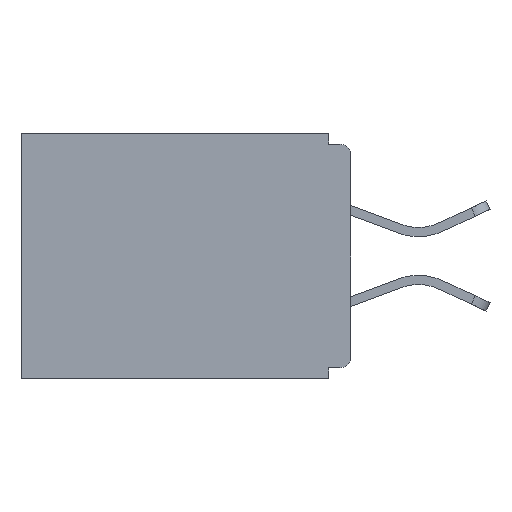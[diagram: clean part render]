
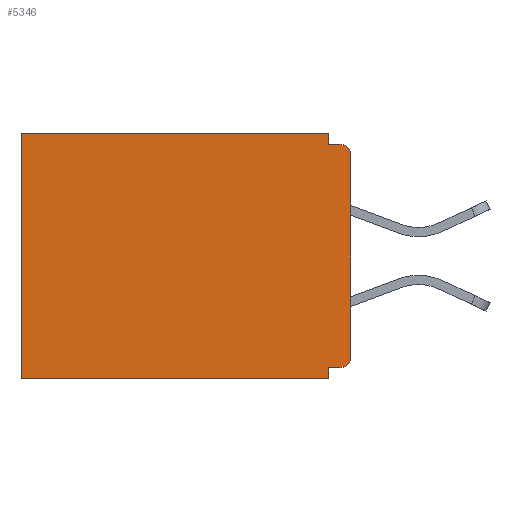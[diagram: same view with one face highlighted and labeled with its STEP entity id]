
A CAD part, left-side view. The second image highlights one B-rep face of the part: STEP entity #5346.
In plain terms, the highlighted planar face has unit normal (-1, 0, 0).
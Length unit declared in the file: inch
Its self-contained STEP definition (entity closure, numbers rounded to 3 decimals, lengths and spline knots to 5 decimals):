
#561 = CARTESIAN_POINT ( 'NONE',  ( 0.298, 0., -0.03 ) ) ;
#940 = VERTEX_POINT ( 'NONE', #1920 ) ;
#970 = VECTOR ( 'NONE', #1471, 39.37008 ) ;
#1181 = DIRECTION ( 'NONE',  ( 0., 0., -1. ) ) ;
#1192 = CARTESIAN_POINT ( 'NONE',  ( 0.298, 0.015, -0.015 ) ) ;
#1256 = DIRECTION ( 'NONE',  ( 0., 0., -1. ) ) ;
#1259 = DIRECTION ( 'NONE',  ( 0., -1., 0. ) ) ;
#1322 = VECTOR ( 'NONE', #5006, 39.37008 ) ;
#1471 = DIRECTION ( 'NONE',  ( 0., 0., -1. ) ) ;
#1920 = CARTESIAN_POINT ( 'NONE',  ( 0.298, 0., -0.313 ) ) ;
#2230 = AXIS2_PLACEMENT_3D ( 'NONE', #13511, #8339, #1256 ) ;
#2332 = EDGE_LOOP ( 'NONE', ( #15983, #18313, #9419, #7935, #17134, #21832, #17767, #9059, #19388, #3299 ) ) ;
#2635 = EDGE_CURVE ( 'NONE', #10745, #18288, #10756, .T. ) ;
#3299 = ORIENTED_EDGE ( 'NONE', *, *, #9171, .F. ) ;
#3429 = DIRECTION ( 'NONE',  ( 0., 0., -1. ) ) ;
#3527 = FACE_OUTER_BOUND ( 'NONE', #2332, .T. ) ;
#3716 = VECTOR ( 'NONE', #15571, 39.37008 ) ;
#3941 = CARTESIAN_POINT ( 'NONE',  ( 0.298, 0.46, -0.343 ) ) ;
#4292 = CARTESIAN_POINT ( 'NONE',  ( 0.298, 0.031, -0.343 ) ) ;
#4934 = CARTESIAN_POINT ( 'NONE',  ( 0.298, 0.015, -0.03 ) ) ;
#4982 = CIRCLE ( 'NONE', #10778, 0.015 ) ;
#5006 = DIRECTION ( 'NONE',  ( 0., 1., 0. ) ) ;
#5346 = ADVANCED_FACE ( 'NONE', ( #3527 ), #20271, .F. ) ;
#5601 = VECTOR ( 'NONE', #10202, 39.37008 ) ;
#5848 = LINE ( 'NONE', #20559, #5601 ) ;
#6840 = CARTESIAN_POINT ( 'NONE',  ( 0.298, 0., 0. ) ) ;
#7559 = LINE ( 'NONE', #6840, #11602 ) ;
#7646 = VERTEX_POINT ( 'NONE', #9323 ) ;
#7935 = ORIENTED_EDGE ( 'NONE', *, *, #17537, .T. ) ;
#8339 = DIRECTION ( 'NONE',  ( 1., 0., 0. ) ) ;
#8606 = CARTESIAN_POINT ( 'NONE',  ( 0.298, 0.031, -0.343 ) ) ;
#8850 = CARTESIAN_POINT ( 'NONE',  ( 0.298, 0.031, -0.015 ) ) ;
#9059 = ORIENTED_EDGE ( 'NONE', *, *, #17984, .F. ) ;
#9065 = LINE ( 'NONE', #11633, #970 ) ;
#9171 = EDGE_CURVE ( 'NONE', #16404, #940, #9065, .T. ) ;
#9214 = CIRCLE ( 'NONE', #11218, 0.015 ) ;
#9238 = DIRECTION ( 'NONE',  ( 0., 0., -1. ) ) ;
#9320 = VECTOR ( 'NONE', #9238, 39.37008 ) ;
#9323 = CARTESIAN_POINT ( 'NONE',  ( 0.298, 0.031, -0.328 ) ) ;
#9419 = ORIENTED_EDGE ( 'NONE', *, *, #13753, .F. ) ;
#10105 = DIRECTION ( 'NONE',  ( 0., 1., 0. ) ) ;
#10187 = EDGE_CURVE ( 'NONE', #7646, #10433, #12568, .T. ) ;
#10202 = DIRECTION ( 'NONE',  ( 0., 1., 0. ) ) ;
#10298 = CARTESIAN_POINT ( 'NONE',  ( 0.298, 0.031, 0. ) ) ;
#10433 = VERTEX_POINT ( 'NONE', #8606 ) ;
#10745 = VERTEX_POINT ( 'NONE', #20727 ) ;
#10756 = LINE ( 'NONE', #13740, #3716 ) ;
#10778 = AXIS2_PLACEMENT_3D ( 'NONE', #20349, #13433, #1181 ) ;
#11218 = AXIS2_PLACEMENT_3D ( 'NONE', #4934, #13816, #3429 ) ;
#11602 = VECTOR ( 'NONE', #10105, 39.37008 ) ;
#11633 = CARTESIAN_POINT ( 'NONE',  ( 0.298, 0., 0. ) ) ;
#12568 = LINE ( 'NONE', #4292, #9320 ) ;
#13433 = DIRECTION ( 'NONE',  ( -1., 0., 0. ) ) ;
#13511 = CARTESIAN_POINT ( 'NONE',  ( 0.298, 0., 0. ) ) ;
#13696 = VERTEX_POINT ( 'NONE', #8850 ) ;
#13740 = CARTESIAN_POINT ( 'NONE',  ( 0.298, 0.46, 0. ) ) ;
#13753 = EDGE_CURVE ( 'NONE', #21129, #13696, #17536, .T. ) ;
#13816 = DIRECTION ( 'NONE',  ( -1., 0., 0. ) ) ;
#14336 = DIRECTION ( 'NONE',  ( 0., 0., -1. ) ) ;
#14561 = VECTOR ( 'NONE', #14336, 39.37008 ) ;
#15040 = CARTESIAN_POINT ( 'NONE',  ( 0.298, 0., -0.015 ) ) ;
#15349 = LINE ( 'NONE', #21942, #1322 ) ;
#15571 = DIRECTION ( 'NONE',  ( 0., 0., -1. ) ) ;
#15983 = ORIENTED_EDGE ( 'NONE', *, *, #22010, .T. ) ;
#16233 = EDGE_CURVE ( 'NONE', #10433, #18288, #5848, .T. ) ;
#16404 = VERTEX_POINT ( 'NONE', #561 ) ;
#16675 = LINE ( 'NONE', #15040, #21061 ) ;
#17134 = ORIENTED_EDGE ( 'NONE', *, *, #2635, .T. ) ;
#17536 = LINE ( 'NONE', #21256, #14561 ) ;
#17537 = EDGE_CURVE ( 'NONE', #21129, #10745, #7559, .T. ) ;
#17767 = ORIENTED_EDGE ( 'NONE', *, *, #10187, .F. ) ;
#17984 = EDGE_CURVE ( 'NONE', #21777, #7646, #15349, .T. ) ;
#18004 = EDGE_CURVE ( 'NONE', #13696, #19732, #16675, .T. ) ;
#18288 = VERTEX_POINT ( 'NONE', #3941 ) ;
#18313 = ORIENTED_EDGE ( 'NONE', *, *, #18004, .F. ) ;
#19388 = ORIENTED_EDGE ( 'NONE', *, *, #20104, .T. ) ;
#19732 = VERTEX_POINT ( 'NONE', #1192 ) ;
#20104 = EDGE_CURVE ( 'NONE', #21777, #940, #4982, .T. ) ;
#20271 = PLANE ( 'NONE',  #2230 ) ;
#20349 = CARTESIAN_POINT ( 'NONE',  ( 0.298, 0.015, -0.313 ) ) ;
#20559 = CARTESIAN_POINT ( 'NONE',  ( 0.298, 0., -0.343 ) ) ;
#20727 = CARTESIAN_POINT ( 'NONE',  ( 0.298, 0.46, 0. ) ) ;
#21061 = VECTOR ( 'NONE', #1259, 39.37008 ) ;
#21129 = VERTEX_POINT ( 'NONE', #10298 ) ;
#21256 = CARTESIAN_POINT ( 'NONE',  ( 0.298, 0.031, -0.343 ) ) ;
#21436 = CARTESIAN_POINT ( 'NONE',  ( 0.298, 0.015, -0.328 ) ) ;
#21777 = VERTEX_POINT ( 'NONE', #21436 ) ;
#21832 = ORIENTED_EDGE ( 'NONE', *, *, #16233, .F. ) ;
#21942 = CARTESIAN_POINT ( 'NONE',  ( 0.298, 0., -0.328 ) ) ;
#22010 = EDGE_CURVE ( 'NONE', #16404, #19732, #9214, .T. ) ;
